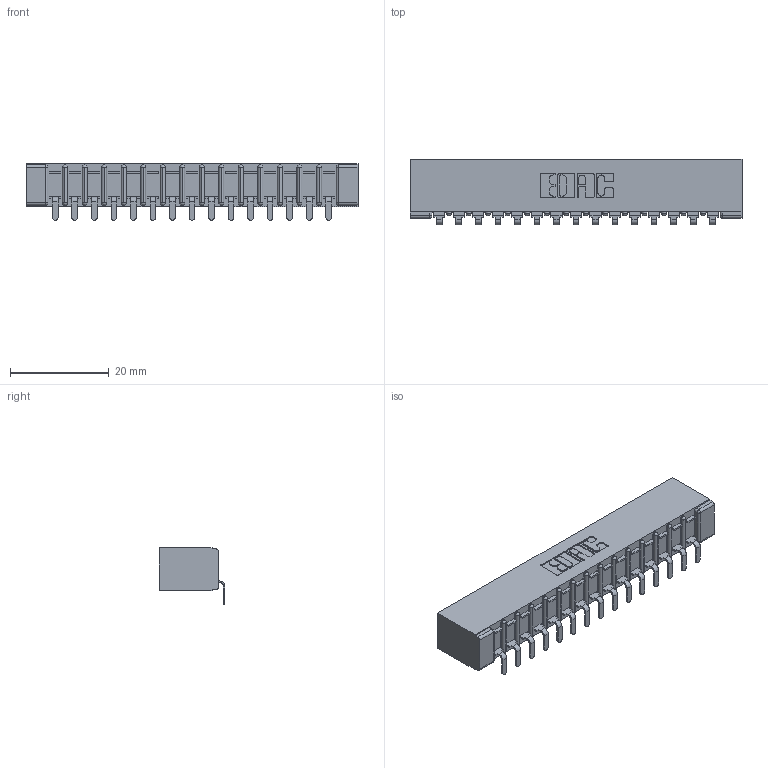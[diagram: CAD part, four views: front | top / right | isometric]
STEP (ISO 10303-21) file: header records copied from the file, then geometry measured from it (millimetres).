
FILE_DESCRIPTION (( 'STEP AP203' ), '1' );
FILE_NAME ('357-015-553-101.STEP', '2018-08-08T01:25:48', ( '' ), ( '' ), 'SwSTEP 2.0', 'SolidWorks 2016', '' );
FILE_SCHEMA (( 'CONFIG_CONTROL_DESIGN' ));
Length unit declared in the file: inch
Products named in the file (3): 307 Part_No Mounting Lugs; 307-290-002_553; 357-015-553-101
Assembly tree (16 placements, depth 2):
  357-015-553-101
    307 Part_No Mounting Lugs
    307-290-002_553  x15
Bounding box: 67.31 x 13.32 x 11.51 mm (x, y, z)
Volume: 4682.2 mm3; surface area: 8638.8 mm2
Topology: 16 solids, 16 shells, 1296 faces, 3959 edges, 2594 vertices
Faces by surface type: plane 771, cylinder 493, sphere 32
Entity records: 16764 total; most frequent: CARTESIAN_POINT 2824, ORIENTED_EDGE 2814, DIRECTION 2755, EDGE_CURVE 1407, VECTOR 1065, LINE 1065, VERTEX_POINT 914, AXIS2_PLACEMENT_3D 845
